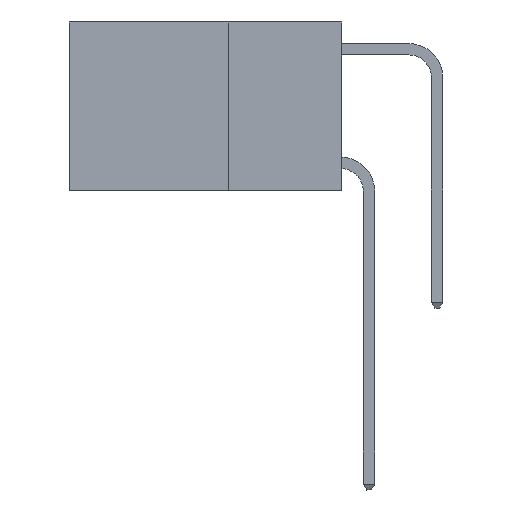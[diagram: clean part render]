
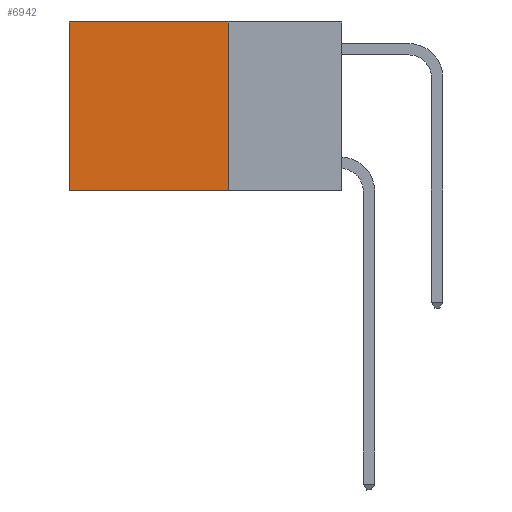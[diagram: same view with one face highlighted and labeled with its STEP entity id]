
A CAD part, left-side view. The second image highlights one B-rep face of the part: STEP entity #6942.
In plain terms, the highlighted planar face has unit normal (-1, 0, 0).
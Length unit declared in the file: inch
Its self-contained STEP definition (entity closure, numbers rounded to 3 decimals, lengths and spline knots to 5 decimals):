
#289 = VECTOR ( 'NONE', #1856, 39.37008 ) ;
#714 = DIRECTION ( 'NONE',  ( 0., 0., -1. ) ) ;
#1856 = DIRECTION ( 'NONE',  ( 0., 0., -1. ) ) ;
#2696 = ORIENTED_EDGE ( 'NONE', *, *, #10857, .F. ) ;
#3358 = CARTESIAN_POINT ( 'NONE',  ( 0.2625, 0.25, -0.37 ) ) ;
#4649 = VERTEX_POINT ( 'NONE', #6718 ) ;
#5266 = CARTESIAN_POINT ( 'NONE',  ( 0.2625, 0.25, 0. ) ) ;
#5665 = DIRECTION ( 'NONE',  ( 0., 0., -1. ) ) ;
#6718 = CARTESIAN_POINT ( 'NONE',  ( 0.2625, 0.6, 0. ) ) ;
#6942 = ADVANCED_FACE ( 'NONE', ( #17838 ), #6986, .F. ) ;
#6986 = PLANE ( 'NONE',  #13592 ) ;
#7132 = CARTESIAN_POINT ( 'NONE',  ( 0.2625, 0.25, 0. ) ) ;
#7289 = EDGE_CURVE ( 'NONE', #16443, #9264, #19209, .T. ) ;
#7539 = EDGE_CURVE ( 'NONE', #16443, #4649, #12106, .T. ) ;
#9264 = VERTEX_POINT ( 'NONE', #9544 ) ;
#9544 = CARTESIAN_POINT ( 'NONE',  ( 0.2625, 0.25, -0.37 ) ) ;
#9575 = ORIENTED_EDGE ( 'NONE', *, *, #7289, .F. ) ;
#9666 = LINE ( 'NONE', #11497, #15186 ) ;
#10857 = EDGE_CURVE ( 'NONE', #9264, #13122, #17661, .T. ) ;
#11202 = CARTESIAN_POINT ( 'NONE',  ( 0.2625, 0.25, 0. ) ) ;
#11446 = VECTOR ( 'NONE', #12695, 39.37008 ) ;
#11497 = CARTESIAN_POINT ( 'NONE',  ( 0.2625, 0.6, 0. ) ) ;
#12106 = LINE ( 'NONE', #15248, #17175 ) ;
#12695 = DIRECTION ( 'NONE',  ( 0., 1., 0. ) ) ;
#13122 = VERTEX_POINT ( 'NONE', #14233 ) ;
#13592 = AXIS2_PLACEMENT_3D ( 'NONE', #5266, #14695, #5665 ) ;
#14233 = CARTESIAN_POINT ( 'NONE',  ( 0.2625, 0.6, -0.37 ) ) ;
#14406 = EDGE_LOOP ( 'NONE', ( #18564, #2696, #9575, #16501 ) ) ;
#14695 = DIRECTION ( 'NONE',  ( 1., 0., 0. ) ) ;
#15186 = VECTOR ( 'NONE', #714, 39.37008 ) ;
#15248 = CARTESIAN_POINT ( 'NONE',  ( 0.2625, 0.25, 0. ) ) ;
#15443 = DIRECTION ( 'NONE',  ( 0., 1., 0. ) ) ;
#16443 = VERTEX_POINT ( 'NONE', #7132 ) ;
#16501 = ORIENTED_EDGE ( 'NONE', *, *, #7539, .T. ) ;
#17129 = EDGE_CURVE ( 'NONE', #4649, #13122, #9666, .T. ) ;
#17175 = VECTOR ( 'NONE', #15443, 39.37008 ) ;
#17661 = LINE ( 'NONE', #3358, #11446 ) ;
#17838 = FACE_OUTER_BOUND ( 'NONE', #14406, .T. ) ;
#18564 = ORIENTED_EDGE ( 'NONE', *, *, #17129, .T. ) ;
#19209 = LINE ( 'NONE', #11202, #289 ) ;
